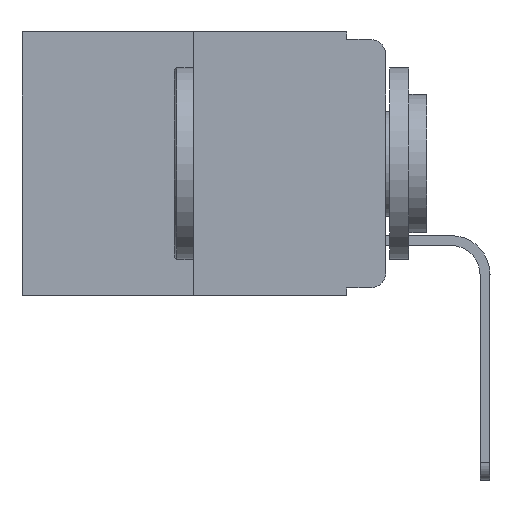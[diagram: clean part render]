
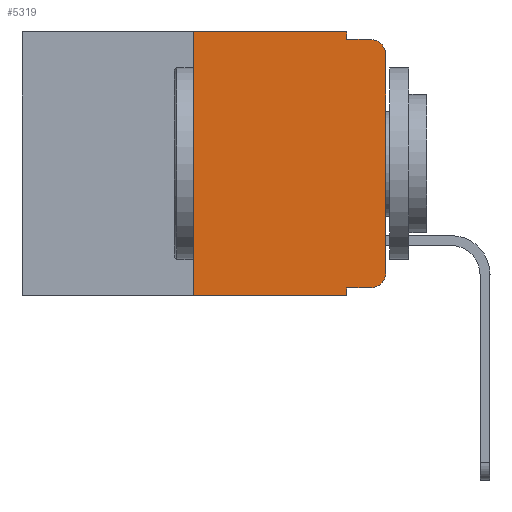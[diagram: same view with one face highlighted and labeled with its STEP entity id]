
A CAD part, left-side view. The second image highlights one B-rep face of the part: STEP entity #5319.
In plain terms, the highlighted planar face has unit normal (-1, 0, 0).
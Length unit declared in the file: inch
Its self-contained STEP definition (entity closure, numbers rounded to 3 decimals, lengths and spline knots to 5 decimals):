
#271 = DIRECTION ( 'NONE',  ( 0., 0., -1. ) ) ;
#564 = CARTESIAN_POINT ( 'NONE',  ( 0., 0.051, 0. ) ) ;
#754 = DIRECTION ( 'NONE',  ( 0., 0., -1. ) ) ;
#827 = AXIS2_PLACEMENT_3D ( 'NONE', #3765, #3689, #6912 ) ;
#1138 = CIRCLE ( 'NONE', #827, 0.02 ) ;
#1317 = VECTOR ( 'NONE', #8048, 39.37008 ) ;
#1439 = LINE ( 'NONE', #564, #14211 ) ;
#2642 = EDGE_CURVE ( 'NONE', #15591, #8323, #1439, .T. ) ;
#2766 = CARTESIAN_POINT ( 'NONE',  ( 0., 0.051, -0.343 ) ) ;
#3151 = ORIENTED_EDGE ( 'NONE', *, *, #8001, .T. ) ;
#3245 = ORIENTED_EDGE ( 'NONE', *, *, #5032, .F. ) ;
#3305 = VECTOR ( 'NONE', #9025, 39.37008 ) ;
#3500 = EDGE_CURVE ( 'NONE', #16287, #15591, #17006, .T. ) ;
#3689 = DIRECTION ( 'NONE',  ( -1., 0., 0. ) ) ;
#3741 = DIRECTION ( 'NONE',  ( 0., 0., 1. ) ) ;
#3765 = CARTESIAN_POINT ( 'NONE',  ( 0., 0.02, -0.03 ) ) ;
#3935 = ORIENTED_EDGE ( 'NONE', *, *, #2642, .F. ) ;
#4417 = VERTEX_POINT ( 'NONE', #6509 ) ;
#4637 = EDGE_CURVE ( 'NONE', #15318, #15475, #14770, .T. ) ;
#4961 = CARTESIAN_POINT ( 'NONE',  ( 0., 0.25, 0. ) ) ;
#5032 = EDGE_CURVE ( 'NONE', #8323, #10295, #19890, .T. ) ;
#5319 = ADVANCED_FACE ( 'NONE', ( #14733 ), #20104, .F. ) ;
#5371 = CARTESIAN_POINT ( 'NONE',  ( 0., 0.25, -0.343 ) ) ;
#5443 = CARTESIAN_POINT ( 'NONE',  ( 0., 0., 0. ) ) ;
#5849 = DIRECTION ( 'NONE',  ( 0., 0., -1. ) ) ;
#5883 = VECTOR ( 'NONE', #3741, 39.37008 ) ;
#6020 = ORIENTED_EDGE ( 'NONE', *, *, #10355, .T. ) ;
#6080 = CARTESIAN_POINT ( 'NONE',  ( 0., 0.051, -0.333 ) ) ;
#6509 = CARTESIAN_POINT ( 'NONE',  ( 0., 0.051, -0.333 ) ) ;
#6816 = ORIENTED_EDGE ( 'NONE', *, *, #12188, .T. ) ;
#6912 = DIRECTION ( 'NONE',  ( 0., 0., -1. ) ) ;
#7075 = CARTESIAN_POINT ( 'NONE',  ( 0., 0., -0.313 ) ) ;
#7108 = ORIENTED_EDGE ( 'NONE', *, *, #4637, .T. ) ;
#7853 = CARTESIAN_POINT ( 'NONE',  ( 0., 0.051, 0. ) ) ;
#8001 = EDGE_CURVE ( 'NONE', #12259, #10295, #1138, .T. ) ;
#8048 = DIRECTION ( 'NONE',  ( 0., -1., 0. ) ) ;
#8211 = ORIENTED_EDGE ( 'NONE', *, *, #16446, .F. ) ;
#8318 = LINE ( 'NONE', #7853, #16168 ) ;
#8323 = VERTEX_POINT ( 'NONE', #16985 ) ;
#8359 = VECTOR ( 'NONE', #11549, 39.37008 ) ;
#8929 = CARTESIAN_POINT ( 'NONE',  ( 0., 0.051, 0. ) ) ;
#9025 = DIRECTION ( 'NONE',  ( 0., -1., 0. ) ) ;
#9192 = AXIS2_PLACEMENT_3D ( 'NONE', #13826, #18491, #5849 ) ;
#9194 = ORIENTED_EDGE ( 'NONE', *, *, #18839, .T. ) ;
#9436 = ORIENTED_EDGE ( 'NONE', *, *, #3500, .F. ) ;
#9767 = CARTESIAN_POINT ( 'NONE',  ( 0., 0.473, -0.343 ) ) ;
#9891 = CARTESIAN_POINT ( 'NONE',  ( 0., 0.02, -0.01 ) ) ;
#10295 = VERTEX_POINT ( 'NONE', #9891 ) ;
#10329 = EDGE_LOOP ( 'NONE', ( #6020, #3151, #3245, #3935, #9436, #13089, #6816, #8211, #9194, #7108 ) ) ;
#10355 = EDGE_CURVE ( 'NONE', #15475, #12259, #18412, .T. ) ;
#10398 = LINE ( 'NONE', #6080, #3305 ) ;
#10731 = CARTESIAN_POINT ( 'NONE',  ( 0., 0.25, 0. ) ) ;
#11345 = VECTOR ( 'NONE', #15932, 39.37008 ) ;
#11537 = CARTESIAN_POINT ( 'NONE',  ( 0., 0.02, -0.333 ) ) ;
#11549 = DIRECTION ( 'NONE',  ( 0., -1., 0. ) ) ;
#12188 = EDGE_CURVE ( 'NONE', #19224, #13234, #14887, .T. ) ;
#12259 = VERTEX_POINT ( 'NONE', #17752 ) ;
#13089 = ORIENTED_EDGE ( 'NONE', *, *, #15249, .F. ) ;
#13152 = AXIS2_PLACEMENT_3D ( 'NONE', #19488, #14813, #754 ) ;
#13234 = VERTEX_POINT ( 'NONE', #2766 ) ;
#13826 = CARTESIAN_POINT ( 'NONE',  ( 0., 0.473, 0. ) ) ;
#14211 = VECTOR ( 'NONE', #17905, 39.37008 ) ;
#14733 = FACE_OUTER_BOUND ( 'NONE', #10329, .T. ) ;
#14770 = CIRCLE ( 'NONE', #13152, 0.02 ) ;
#14813 = DIRECTION ( 'NONE',  ( -1., 0., 0. ) ) ;
#14887 = LINE ( 'NONE', #9767, #16846 ) ;
#15249 = EDGE_CURVE ( 'NONE', #19224, #16287, #15527, .T. ) ;
#15318 = VERTEX_POINT ( 'NONE', #11537 ) ;
#15475 = VERTEX_POINT ( 'NONE', #7075 ) ;
#15527 = LINE ( 'NONE', #4961, #11345 ) ;
#15591 = VERTEX_POINT ( 'NONE', #8929 ) ;
#15932 = DIRECTION ( 'NONE',  ( 0., 0., 1. ) ) ;
#16009 = CARTESIAN_POINT ( 'NONE',  ( 0., 0.051, -0.01 ) ) ;
#16168 = VECTOR ( 'NONE', #271, 39.37008 ) ;
#16287 = VERTEX_POINT ( 'NONE', #10731 ) ;
#16446 = EDGE_CURVE ( 'NONE', #4417, #13234, #8318, .T. ) ;
#16846 = VECTOR ( 'NONE', #19130, 39.37008 ) ;
#16985 = CARTESIAN_POINT ( 'NONE',  ( 0., 0.051, -0.01 ) ) ;
#17006 = LINE ( 'NONE', #17656, #1317 ) ;
#17656 = CARTESIAN_POINT ( 'NONE',  ( 0., 0.473, 0. ) ) ;
#17752 = CARTESIAN_POINT ( 'NONE',  ( 0., 0., -0.03 ) ) ;
#17905 = DIRECTION ( 'NONE',  ( 0., 0., -1. ) ) ;
#18412 = LINE ( 'NONE', #5443, #5883 ) ;
#18491 = DIRECTION ( 'NONE',  ( 1., 0., 0. ) ) ;
#18839 = EDGE_CURVE ( 'NONE', #4417, #15318, #10398, .T. ) ;
#19130 = DIRECTION ( 'NONE',  ( 0., -1., 0. ) ) ;
#19224 = VERTEX_POINT ( 'NONE', #5371 ) ;
#19488 = CARTESIAN_POINT ( 'NONE',  ( 0., 0.02, -0.313 ) ) ;
#19890 = LINE ( 'NONE', #16009, #8359 ) ;
#20104 = PLANE ( 'NONE',  #9192 ) ;
